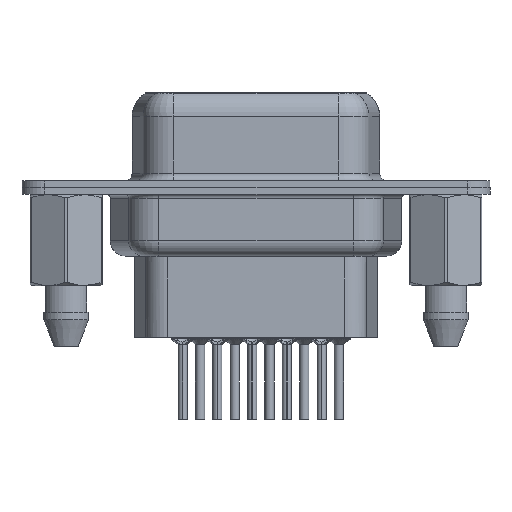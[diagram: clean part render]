
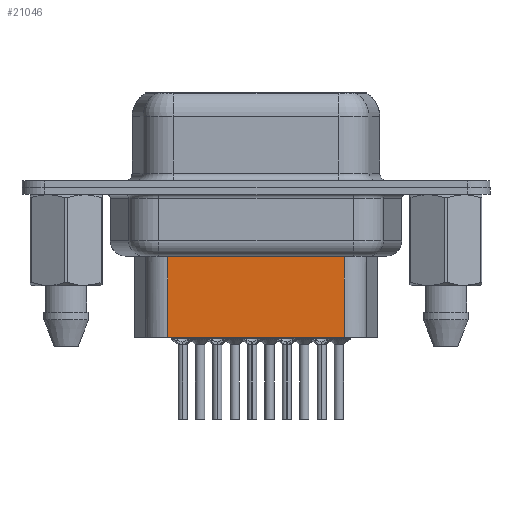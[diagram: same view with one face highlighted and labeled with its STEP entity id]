
A CAD part, front view. The second image highlights one B-rep face of the part: STEP entity #21046.
In plain terms, the highlighted planar face has unit normal (0, -1, 0).
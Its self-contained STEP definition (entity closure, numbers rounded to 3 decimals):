
#377 = ORIENTED_EDGE ( 'NONE', *, *, #495, .T. ) ;
#495 = EDGE_CURVE ( 'NONE', #8053, #17926, #5754, .T. ) ;
#1362 = DIRECTION ( 'NONE',  ( 1., 0., 0. ) ) ;
#3198 = CARTESIAN_POINT ( 'NONE',  ( 6.701, -3.5, -4.097 ) ) ;
#3768 = DIRECTION ( 'NONE',  ( 0., 0., -1. ) ) ;
#5744 = CARTESIAN_POINT ( 'NONE',  ( 6.701, -3.5, -9.85 ) ) ;
#5754 = LINE ( 'NONE', #19667, #11050 ) ;
#6276 = LINE ( 'NONE', #19813, #17655 ) ;
#6562 = ORIENTED_EDGE ( 'NONE', *, *, #25300, .F. ) ;
#7443 = CARTESIAN_POINT ( 'NONE',  ( 18.289, -3.5, -4.097 ) ) ;
#8053 = VERTEX_POINT ( 'NONE', #3198 ) ;
#8166 = EDGE_CURVE ( 'NONE', #10772, #17926, #23499, .T. ) ;
#8364 = CARTESIAN_POINT ( 'NONE',  ( 6.701, -3.5, -9.85 ) ) ;
#8462 = DIRECTION ( 'NONE',  ( -1., 0., 0. ) ) ;
#9215 = VECTOR ( 'NONE', #25745, 1000. ) ;
#9836 = CARTESIAN_POINT ( 'NONE',  ( 18.289, -3.5, -3.1 ) ) ;
#10772 = VERTEX_POINT ( 'NONE', #26224 ) ;
#11050 = VECTOR ( 'NONE', #3768, 1000. ) ;
#14569 = LINE ( 'NONE', #9836, #9215 ) ;
#14629 = VERTEX_POINT ( 'NONE', #7443 ) ;
#14868 = PLANE ( 'NONE',  #27682 ) ;
#14959 = DIRECTION ( 'NONE',  ( 0., -1., 0. ) ) ;
#17274 = EDGE_LOOP ( 'NONE', ( #6562, #29058, #377, #26248 ) ) ;
#17570 = FACE_OUTER_BOUND ( 'NONE', #17274, .T. ) ;
#17655 = VECTOR ( 'NONE', #8462, 1000. ) ;
#17926 = VERTEX_POINT ( 'NONE', #5744 ) ;
#18878 = VECTOR ( 'NONE', #24175, 1000. ) ;
#19003 = EDGE_CURVE ( 'NONE', #14629, #8053, #6276, .T. ) ;
#19667 = CARTESIAN_POINT ( 'NONE',  ( 6.701, -3.5, -3.1 ) ) ;
#19813 = CARTESIAN_POINT ( 'NONE',  ( 6.454, -3.5, -4.097 ) ) ;
#21046 = ADVANCED_FACE ( 'NONE', ( #17570 ), #14868, .T. ) ;
#23499 = LINE ( 'NONE', #8364, #18878 ) ;
#24175 = DIRECTION ( 'NONE',  ( -1., 0., 0. ) ) ;
#25300 = EDGE_CURVE ( 'NONE', #14629, #10772, #14569, .T. ) ;
#25745 = DIRECTION ( 'NONE',  ( 0., 0., -1. ) ) ;
#26224 = CARTESIAN_POINT ( 'NONE',  ( 18.289, -3.5, -9.85 ) ) ;
#26248 = ORIENTED_EDGE ( 'NONE', *, *, #8166, .F. ) ;
#27682 = AXIS2_PLACEMENT_3D ( 'NONE', #28580, #14959, #1362 ) ;
#28580 = CARTESIAN_POINT ( 'NONE',  ( 6.701, -3.5, -3.1 ) ) ;
#29058 = ORIENTED_EDGE ( 'NONE', *, *, #19003, .T. ) ;
